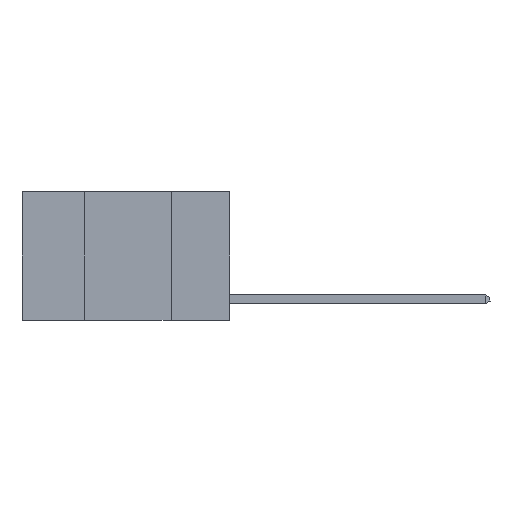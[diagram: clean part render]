
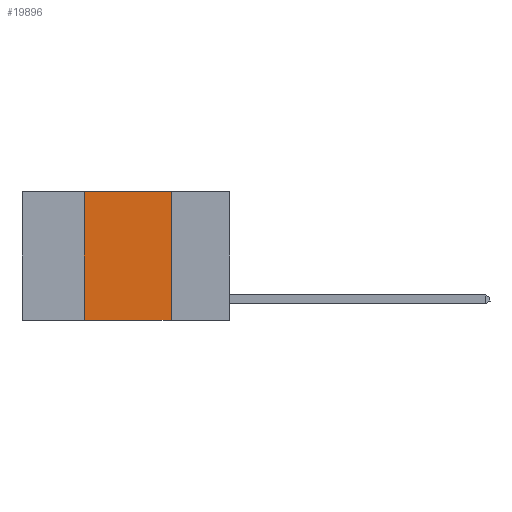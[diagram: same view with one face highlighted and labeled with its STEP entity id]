
A CAD part, left-side view. The second image highlights one B-rep face of the part: STEP entity #19896.
In plain terms, the highlighted planar face has unit normal (-1, 0, 0).
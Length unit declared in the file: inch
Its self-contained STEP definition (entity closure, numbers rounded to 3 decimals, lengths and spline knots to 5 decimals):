
#1012 = ORIENTED_EDGE ( 'NONE', *, *, #10995, .F. ) ;
#2191 = CARTESIAN_POINT ( 'NONE',  ( 0., 0.42, -0.37 ) ) ;
#2201 = CARTESIAN_POINT ( 'NONE',  ( 0., 0.6, -0.37 ) ) ;
#2958 = EDGE_CURVE ( 'NONE', #7580, #11746, #5512, .T. ) ;
#3751 = VECTOR ( 'NONE', #5731, 39.37008 ) ;
#4280 = DIRECTION ( 'NONE',  ( 1., 0., 0. ) ) ;
#4390 = CARTESIAN_POINT ( 'NONE',  ( 0., 0.42, 0. ) ) ;
#5512 = LINE ( 'NONE', #2201, #3751 ) ;
#5731 = DIRECTION ( 'NONE',  ( 0., -1., 0. ) ) ;
#6061 = VECTOR ( 'NONE', #18224, 39.37008 ) ;
#6162 = PLANE ( 'NONE',  #14249 ) ;
#6275 = FACE_OUTER_BOUND ( 'NONE', #8492, .T. ) ;
#7052 = ORIENTED_EDGE ( 'NONE', *, *, #19752, .F. ) ;
#7580 = VERTEX_POINT ( 'NONE', #2191 ) ;
#8492 = EDGE_LOOP ( 'NONE', ( #7052, #13677, #1012, #11307 ) ) ;
#9576 = LINE ( 'NONE', #21407, #6061 ) ;
#10020 = VECTOR ( 'NONE', #18754, 39.37008 ) ;
#10901 = CARTESIAN_POINT ( 'NONE',  ( 0., 0.42, 0. ) ) ;
#10903 = LINE ( 'NONE', #4390, #16504 ) ;
#10995 = EDGE_CURVE ( 'NONE', #7580, #12630, #10903, .T. ) ;
#11307 = ORIENTED_EDGE ( 'NONE', *, *, #2958, .T. ) ;
#11746 = VERTEX_POINT ( 'NONE', #17253 ) ;
#12546 = DIRECTION ( 'NONE',  ( 0., 0., 1. ) ) ;
#12630 = VERTEX_POINT ( 'NONE', #10901 ) ;
#13677 = ORIENTED_EDGE ( 'NONE', *, *, #14396, .F. ) ;
#14097 = CARTESIAN_POINT ( 'NONE',  ( 0., 0.17, 0. ) ) ;
#14249 = AXIS2_PLACEMENT_3D ( 'NONE', #17646, #4280, #18086 ) ;
#14396 = EDGE_CURVE ( 'NONE', #12630, #15499, #9576, .T. ) ;
#15499 = VERTEX_POINT ( 'NONE', #17902 ) ;
#16504 = VECTOR ( 'NONE', #12546, 39.37008 ) ;
#17253 = CARTESIAN_POINT ( 'NONE',  ( 0., 0.17, -0.37 ) ) ;
#17646 = CARTESIAN_POINT ( 'NONE',  ( 0., 0.6, 0. ) ) ;
#17902 = CARTESIAN_POINT ( 'NONE',  ( 0., 0.17, 0. ) ) ;
#18086 = DIRECTION ( 'NONE',  ( 0., 0., -1. ) ) ;
#18224 = DIRECTION ( 'NONE',  ( 0., -1., 0. ) ) ;
#18754 = DIRECTION ( 'NONE',  ( 0., 0., -1. ) ) ;
#19752 = EDGE_CURVE ( 'NONE', #15499, #11746, #20398, .T. ) ;
#19896 = ADVANCED_FACE ( 'NONE', ( #6275 ), #6162, .F. ) ;
#20398 = LINE ( 'NONE', #14097, #10020 ) ;
#21407 = CARTESIAN_POINT ( 'NONE',  ( 0., 0.6, 0. ) ) ;
